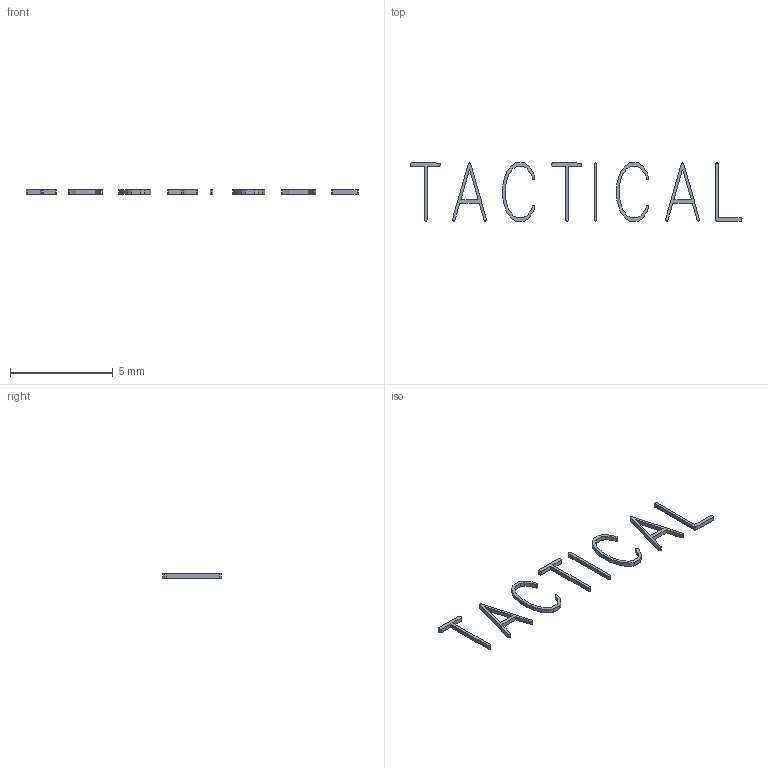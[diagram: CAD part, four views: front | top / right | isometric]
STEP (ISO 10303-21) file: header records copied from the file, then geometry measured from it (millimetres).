
FILE_DESCRIPTION (( 'STEP AP214' ), '1' );
FILE_NAME ('ENGRAVING FILL - TACTICAL.STEP', '2013-06-19T14:03:51', ( 'Asher' ), ( '' ), 'SwSTEP 2.0', 'SolidWorks 2013', '' );
FILE_SCHEMA (( 'AUTOMOTIVE_DESIGN' ));
Length unit declared in the file: millimetre
Products named in the file (1): ENGRAVING FILL - TACTICAL
Bounding box: 16.13 x 2.83 x 0.2 mm (x, y, z)
Volume: 1.1 mm3; surface area: 27.1 mm2
Topology: 8 solids, 8 shells, 177 faces, 483 edges, 322 vertices
Faces by surface type: plane 120, bspline 57
Entity records: 6560 total; most frequent: CARTESIAN_POINT 2360, ORIENTED_EDGE 966, DIRECTION 611, EDGE_CURVE 483, VECTOR 369, LINE 369, VERTEX_POINT 322, EDGE_LOOP 181
